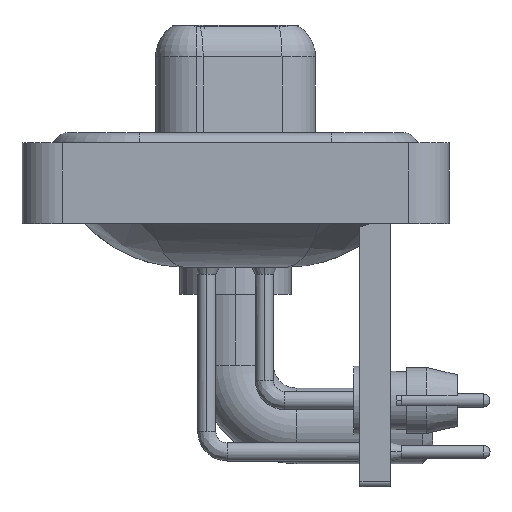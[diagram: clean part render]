
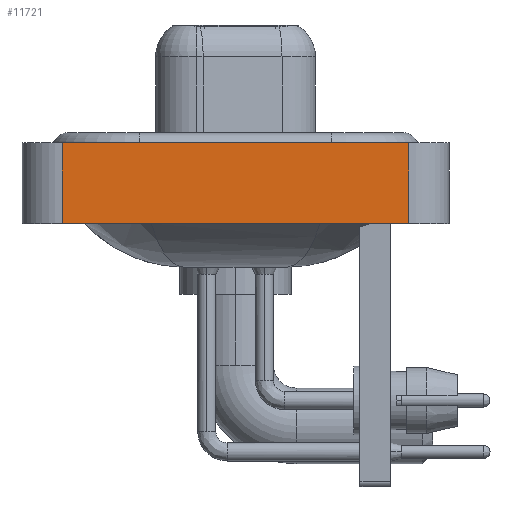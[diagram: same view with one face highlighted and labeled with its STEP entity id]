
A CAD part, left-side view. The second image highlights one B-rep face of the part: STEP entity #11721.
In plain terms, the highlighted planar face has unit normal (-1, 0, 0).
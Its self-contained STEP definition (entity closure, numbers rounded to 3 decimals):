
#769 = DIRECTION ( 'NONE',  ( 0., -1., 0. ) ) ;
#1675 = CARTESIAN_POINT ( 'NONE',  ( -7.25, -8.55, -3.6 ) ) ;
#1679 = VERTEX_POINT ( 'NONE', #19602 ) ;
#1963 = EDGE_CURVE ( 'NONE', #1679, #2871, #20703, .T. ) ;
#2094 = ORIENTED_EDGE ( 'NONE', *, *, #12337, .T. ) ;
#2626 = EDGE_LOOP ( 'NONE', ( #8687, #14761, #9957, #2094 ) ) ;
#2871 = VERTEX_POINT ( 'NONE', #3202 ) ;
#3202 = CARTESIAN_POINT ( 'NONE',  ( -7.25, 8.55, 0.4 ) ) ;
#4640 = VECTOR ( 'NONE', #769, 1000. ) ;
#4830 = VERTEX_POINT ( 'NONE', #21133 ) ;
#5389 = AXIS2_PLACEMENT_3D ( 'NONE', #1675, #8592, #20375 ) ;
#5974 = LINE ( 'NONE', #17770, #4640 ) ;
#6701 = CARTESIAN_POINT ( 'NONE',  ( -7.25, -8.55, -3.6 ) ) ;
#6996 = CARTESIAN_POINT ( 'NONE',  ( -7.25, 8.55, -3.6 ) ) ;
#7799 = VERTEX_POINT ( 'NONE', #6701 ) ;
#8592 = DIRECTION ( 'NONE',  ( -1., 0., 0. ) ) ;
#8687 = ORIENTED_EDGE ( 'NONE', *, *, #19133, .T. ) ;
#9957 = ORIENTED_EDGE ( 'NONE', *, *, #1963, .F. ) ;
#10368 = DIRECTION ( 'NONE',  ( 0., -1., 0. ) ) ;
#11721 = ADVANCED_FACE ( 'NONE', ( #20714 ), #13486, .T. ) ;
#12288 = DIRECTION ( 'NONE',  ( 0., 0., 1. ) ) ;
#12337 = EDGE_CURVE ( 'NONE', #1679, #7799, #5974, .T. ) ;
#13342 = LINE ( 'NONE', #20244, #18726 ) ;
#13486 = PLANE ( 'NONE',  #5389 ) ;
#13576 = DIRECTION ( 'NONE',  ( 0., 0., 1. ) ) ;
#14415 = VECTOR ( 'NONE', #13576, 1000. ) ;
#14761 = ORIENTED_EDGE ( 'NONE', *, *, #18526, .F. ) ;
#17487 = LINE ( 'NONE', #17819, #22207 ) ;
#17770 = CARTESIAN_POINT ( 'NONE',  ( -7.25, -8.55, -3.6 ) ) ;
#17819 = CARTESIAN_POINT ( 'NONE',  ( -7.25, -8.55, -3.6 ) ) ;
#18526 = EDGE_CURVE ( 'NONE', #2871, #4830, #13342, .T. ) ;
#18726 = VECTOR ( 'NONE', #10368, 1000. ) ;
#19133 = EDGE_CURVE ( 'NONE', #7799, #4830, #17487, .T. ) ;
#19602 = CARTESIAN_POINT ( 'NONE',  ( -7.25, 8.55, -3.6 ) ) ;
#20244 = CARTESIAN_POINT ( 'NONE',  ( -7.25, -8.55, 0.4 ) ) ;
#20375 = DIRECTION ( 'NONE',  ( 0., 0., 1. ) ) ;
#20703 = LINE ( 'NONE', #6996, #14415 ) ;
#20714 = FACE_OUTER_BOUND ( 'NONE', #2626, .T. ) ;
#21133 = CARTESIAN_POINT ( 'NONE',  ( -7.25, -8.55, 0.4 ) ) ;
#22207 = VECTOR ( 'NONE', #12288, 1000. ) ;
